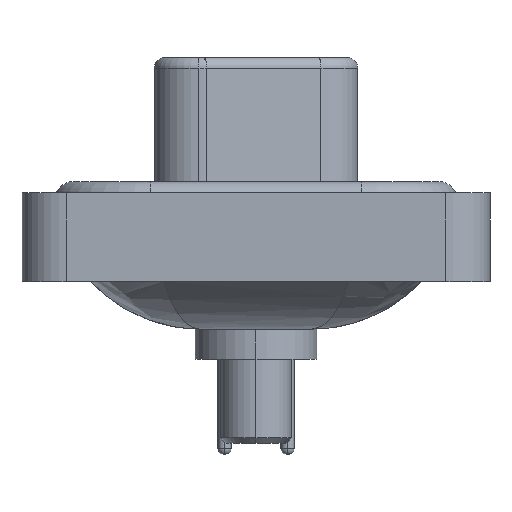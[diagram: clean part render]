
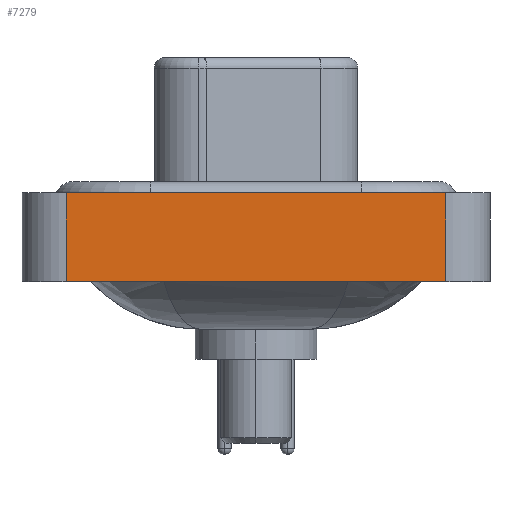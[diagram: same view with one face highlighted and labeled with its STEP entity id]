
A CAD part, left-side view. The second image highlights one B-rep face of the part: STEP entity #7279.
In plain terms, the highlighted planar face has unit normal (-1, 0, 0).
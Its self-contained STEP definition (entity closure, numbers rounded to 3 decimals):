
#265 = EDGE_CURVE ( 'NONE', #20916, #2497, #10202, .T. ) ;
#318 = VECTOR ( 'NONE', #2582, 1000. ) ;
#1676 = DIRECTION ( 'NONE',  ( 0., 0., 1. ) ) ;
#1679 = VECTOR ( 'NONE', #14615, 1000. ) ;
#1840 = DIRECTION ( 'NONE',  ( -1., 0., 0. ) ) ;
#1953 = CARTESIAN_POINT ( 'NONE',  ( -7.35, -8.55, -3.6 ) ) ;
#2277 = DIRECTION ( 'NONE',  ( 0., 0., 1. ) ) ;
#2497 = VERTEX_POINT ( 'NONE', #9973 ) ;
#2582 = DIRECTION ( 'NONE',  ( 0., -1., 0. ) ) ;
#4079 = ORIENTED_EDGE ( 'NONE', *, *, #5079, .T. ) ;
#4140 = LINE ( 'NONE', #9529, #318 ) ;
#4874 = DIRECTION ( 'NONE',  ( 0., -1., 0. ) ) ;
#5079 = EDGE_CURVE ( 'NONE', #16688, #15672, #21206, .T. ) ;
#5898 = EDGE_LOOP ( 'NONE', ( #4079, #13164, #7490, #7860 ) ) ;
#6567 = CARTESIAN_POINT ( 'NONE',  ( -7.35, -8.55, 0.4 ) ) ;
#7279 = ADVANCED_FACE ( 'NONE', ( #10791 ), #12398, .T. ) ;
#7490 = ORIENTED_EDGE ( 'NONE', *, *, #265, .F. ) ;
#7546 = CARTESIAN_POINT ( 'NONE',  ( -7.35, -8.55, -3.6 ) ) ;
#7860 = ORIENTED_EDGE ( 'NONE', *, *, #13511, .T. ) ;
#9529 = CARTESIAN_POINT ( 'NONE',  ( -7.35, -8.55, -3.6 ) ) ;
#9973 = CARTESIAN_POINT ( 'NONE',  ( -7.35, 8.55, 0.4 ) ) ;
#10202 = LINE ( 'NONE', #17039, #16640 ) ;
#10791 = FACE_OUTER_BOUND ( 'NONE', #5898, .T. ) ;
#10845 = VECTOR ( 'NONE', #4874, 1000. ) ;
#12398 = PLANE ( 'NONE',  #13777 ) ;
#13164 = ORIENTED_EDGE ( 'NONE', *, *, #17550, .F. ) ;
#13511 = EDGE_CURVE ( 'NONE', #20916, #16688, #4140, .T. ) ;
#13777 = AXIS2_PLACEMENT_3D ( 'NONE', #1953, #1840, #2277 ) ;
#14615 = DIRECTION ( 'NONE',  ( 0., 0., 1. ) ) ;
#15092 = LINE ( 'NONE', #6567, #10845 ) ;
#15672 = VERTEX_POINT ( 'NONE', #20195 ) ;
#16640 = VECTOR ( 'NONE', #1676, 1000. ) ;
#16688 = VERTEX_POINT ( 'NONE', #18842 ) ;
#17039 = CARTESIAN_POINT ( 'NONE',  ( -7.35, 8.55, -3.6 ) ) ;
#17550 = EDGE_CURVE ( 'NONE', #2497, #15672, #15092, .T. ) ;
#18842 = CARTESIAN_POINT ( 'NONE',  ( -7.35, -8.55, -3.6 ) ) ;
#20195 = CARTESIAN_POINT ( 'NONE',  ( -7.35, -8.55, 0.4 ) ) ;
#20916 = VERTEX_POINT ( 'NONE', #22075 ) ;
#21206 = LINE ( 'NONE', #7546, #1679 ) ;
#22075 = CARTESIAN_POINT ( 'NONE',  ( -7.35, 8.55, -3.6 ) ) ;
